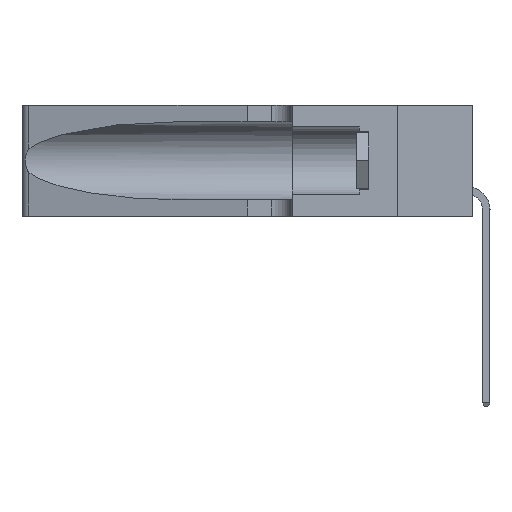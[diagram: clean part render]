
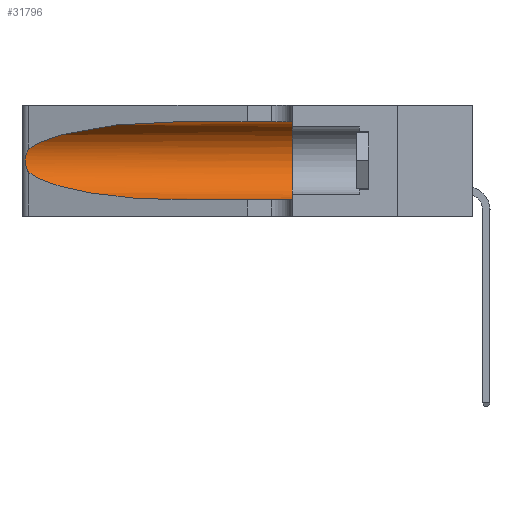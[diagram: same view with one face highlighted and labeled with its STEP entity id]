
A CAD part, left-side view. The second image highlights one B-rep face of the part: STEP entity #31796.
In plain terms, the highlighted cylindrical face has radius 3.308 mm (diameter 6.617 mm), a partial arc.
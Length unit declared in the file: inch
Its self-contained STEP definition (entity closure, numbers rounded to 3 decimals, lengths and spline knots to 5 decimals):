
#495 = CARTESIAN_POINT ( 'NONE',  ( 0.26017, 1.23833, 0.17102 ) ) ;
#603 = CARTESIAN_POINT ( 'NONE',  ( 0.25787, 1.23484, 0.2124 ) ) ;
#2193 = VERTEX_POINT ( 'NONE', #3974 ) ;
#3400 = CARTESIAN_POINT ( 'NONE',  ( 0.1305, 0.35, 0.185 ) ) ;
#3552 = CARTESIAN_POINT ( 'NONE',  ( 0.25789, 1.23486, 0.15765 ) ) ;
#3974 = CARTESIAN_POINT ( 'NONE',  ( 0.1305, 0.72297, 0.31525 ) ) ;
#4775 = ORIENTED_EDGE ( 'NONE', *, *, #34995, .T. ) ;
#4822 = LINE ( 'NONE', #30877, #34781 ) ;
#5291 = VERTEX_POINT ( 'NONE', #35120 ) ;
#5704 = ORIENTED_EDGE ( 'NONE', *, *, #13252, .T. ) ;
#5800 =( BOUNDED_CURVE ( )  B_SPLINE_CURVE ( 3, ( #6864, #21459, #13372, #22104 ),
 .UNSPECIFIED., .F., .T. ) 
 B_SPLINE_CURVE_WITH_KNOTS ( ( 4, 4 ),
 ( 1.5708, 2.84003 ),
 .UNSPECIFIED. ) 
 CURVE ( )  GEOMETRIC_REPRESENTATION_ITEM ( )  RATIONAL_B_SPLINE_CURVE ( ( 1., 0.87, 0.87, 1. ) ) 
 REPRESENTATION_ITEM ( '' )  );
#6252 = ORIENTED_EDGE ( 'NONE', *, *, #22167, .T. ) ;
#6698 = CARTESIAN_POINT ( 'NONE',  ( 0.25487, 1.22718, 0.22369 ) ) ;
#6823 = CARTESIAN_POINT ( 'NONE',  ( 0.26018, 1.23835, 0.19895 ) ) ;
#6864 = CARTESIAN_POINT ( 'NONE',  ( 0.1305, 0.72297, 0.31525 ) ) ;
#7516 = EDGE_LOOP ( 'NONE', ( #5704, #4775, #10014, #6252, #34191, #16044 ) ) ;
#8343 = CARTESIAN_POINT ( 'NONE',  ( 0.1305, 1.61858, 0.185 ) ) ;
#9371 = CARTESIAN_POINT ( 'NONE',  ( 0.26075, 1.23896, 0.178 ) ) ;
#9630 = EDGE_CURVE ( 'NONE', #15701, #34126, #14205, .T. ) ;
#10014 = ORIENTED_EDGE ( 'NONE', *, *, #9630, .T. ) ;
#10654 = DIRECTION ( 'NONE',  ( 0., -1., 0. ) ) ;
#10918 = CIRCLE ( 'NONE', #20887, 0.13025 ) ;
#12069 = EDGE_CURVE ( 'NONE', #2193, #5291, #4822, .T. ) ;
#12280 = CARTESIAN_POINT ( 'NONE',  ( 0.25487, 1.22718, 0.14631 ) ) ;
#13252 = EDGE_CURVE ( 'NONE', #2193, #31981, #5800, .T. ) ;
#13372 = CARTESIAN_POINT ( 'NONE',  ( 0.2373, 1.15595, 0.28018 ) ) ;
#14162 = DIRECTION ( 'NONE',  ( 0., 0., -1. ) ) ;
#14205 =( BOUNDED_CURVE ( )  B_SPLINE_CURVE ( 3, ( #30686, #33873, #18761, #33481 ),
 .UNSPECIFIED., .F., .T. ) 
 B_SPLINE_CURVE_WITH_KNOTS ( ( 4, 4 ),
 ( 3.44316, 4.71239 ),
 .UNSPECIFIED. ) 
 CURVE ( )  GEOMETRIC_REPRESENTATION_ITEM ( )  RATIONAL_B_SPLINE_CURVE ( ( 1., 0.87, 0.87, 1. ) ) 
 REPRESENTATION_ITEM ( '' )  );
#15701 = VERTEX_POINT ( 'NONE', #34527 ) ;
#16044 = ORIENTED_EDGE ( 'NONE', *, *, #12069, .F. ) ;
#18462 = VECTOR ( 'NONE', #10654, 39.37008 ) ;
#18761 = CARTESIAN_POINT ( 'NONE',  ( 0.18966, 0.96281, 0.05475 ) ) ;
#20771 = CARTESIAN_POINT ( 'NONE',  ( 0.25639, 1.23184, 0.21858 ) ) ;
#20887 = AXIS2_PLACEMENT_3D ( 'NONE', #3400, #26116, #23547 ) ;
#21104 = VERTEX_POINT ( 'NONE', #27827 ) ;
#21459 = CARTESIAN_POINT ( 'NONE',  ( 0.18966, 0.96281, 0.31525 ) ) ;
#22104 = CARTESIAN_POINT ( 'NONE',  ( 0.25487, 1.22718, 0.22369 ) ) ;
#22167 = EDGE_CURVE ( 'NONE', #34126, #21104, #23871, .T. ) ;
#23547 = DIRECTION ( 'NONE',  ( 0., 0., 1. ) ) ;
#23695 = CARTESIAN_POINT ( 'NONE',  ( 0.25856, 1.23593, 0.16098 ) ) ;
#23822 = CARTESIAN_POINT ( 'NONE',  ( 0.25639, 1.23186, 0.15144 ) ) ;
#23871 = LINE ( 'NONE', #25006, #18462 ) ;
#24951 = CYLINDRICAL_SURFACE ( 'NONE', #29656, 0.13025 ) ;
#25006 = CARTESIAN_POINT ( 'NONE',  ( 0.1305, 1.61858, 0.05475 ) ) ;
#25809 = CARTESIAN_POINT ( 'NONE',  ( 0.1305, 0.72297, 0.05475 ) ) ;
#26116 = DIRECTION ( 'NONE',  ( 0., 1., 0. ) ) ;
#26748 = CARTESIAN_POINT ( 'NONE',  ( 0.25555, 1.22993, 0.14849 ) ) ;
#27157 = CARTESIAN_POINT ( 'NONE',  ( 0.26075, 1.23896, 0.19203 ) ) ;
#27827 = CARTESIAN_POINT ( 'NONE',  ( 0.1305, 0.35, 0.05475 ) ) ;
#29656 = AXIS2_PLACEMENT_3D ( 'NONE', #8343, #34726, #14162 ) ;
#30686 = CARTESIAN_POINT ( 'NONE',  ( 0.25487, 1.22718, 0.14631 ) ) ;
#30877 = CARTESIAN_POINT ( 'NONE',  ( 0.1305, 1.61858, 0.31525 ) ) ;
#31298 = EDGE_CURVE ( 'NONE', #5291, #21104, #10918, .T. ) ;
#31796 = ADVANCED_FACE ( 'NONE', ( #35349 ), #24951, .F. ) ;
#31981 = VERTEX_POINT ( 'NONE', #35183 ) ;
#33481 = CARTESIAN_POINT ( 'NONE',  ( 0.1305, 0.72297, 0.05475 ) ) ;
#33811 = DIRECTION ( 'NONE',  ( 0., -1., 0. ) ) ;
#33873 = CARTESIAN_POINT ( 'NONE',  ( 0.2373, 1.15595, 0.08982 ) ) ;
#33976 = B_SPLINE_CURVE_WITH_KNOTS ( 'NONE', 3,
 ( #6698, #35752, #20771, #603, #35886, #6823, #27157, #9371, #495, #23695, #3552, #23822, #26748, #12280 ),
 .UNSPECIFIED., .F., .F.,
 ( 4, 2, 2, 2, 2, 2, 4 ),
 ( 0., 0.00027, 0.00053, 0.00107, 0.0016, 0.00187, 0.00214 ),
 .UNSPECIFIED. ) ;
#34126 = VERTEX_POINT ( 'NONE', #25809 ) ;
#34191 = ORIENTED_EDGE ( 'NONE', *, *, #31298, .F. ) ;
#34527 = CARTESIAN_POINT ( 'NONE',  ( 0.25487, 1.22718, 0.14631 ) ) ;
#34726 = DIRECTION ( 'NONE',  ( 0., -1., 0. ) ) ;
#34781 = VECTOR ( 'NONE', #33811, 39.37008 ) ;
#34995 = EDGE_CURVE ( 'NONE', #31981, #15701, #33976, .T. ) ;
#35120 = CARTESIAN_POINT ( 'NONE',  ( 0.1305, 0.35, 0.31525 ) ) ;
#35183 = CARTESIAN_POINT ( 'NONE',  ( 0.25487, 1.22718, 0.22369 ) ) ;
#35349 = FACE_OUTER_BOUND ( 'NONE', #7516, .T. ) ;
#35752 = CARTESIAN_POINT ( 'NONE',  ( 0.25555, 1.22994, 0.2215 ) ) ;
#35886 = CARTESIAN_POINT ( 'NONE',  ( 0.25854, 1.2359, 0.20912 ) ) ;
